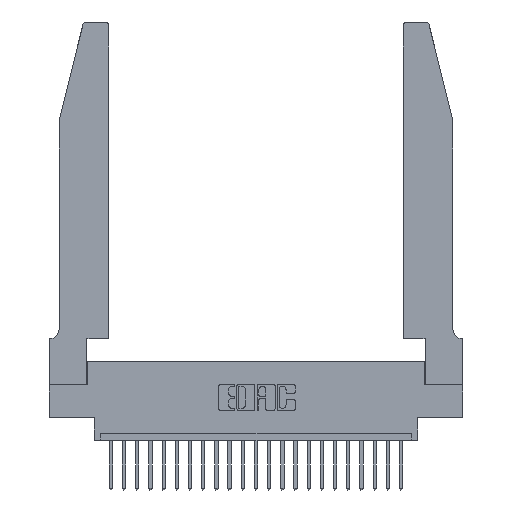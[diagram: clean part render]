
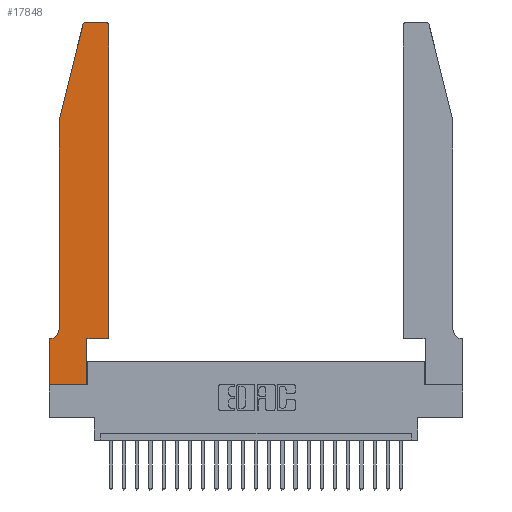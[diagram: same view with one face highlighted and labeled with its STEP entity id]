
A CAD part, top view. The second image highlights one B-rep face of the part: STEP entity #17848.
In plain terms, the highlighted planar face has unit normal (0, 0, 1).
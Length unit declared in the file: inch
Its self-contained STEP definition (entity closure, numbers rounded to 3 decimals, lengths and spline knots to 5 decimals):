
#230 = ORIENTED_EDGE ( 'NONE', *, *, #2061, .T. ) ;
#235 = EDGE_CURVE ( 'NONE', #24340, #12330, #18256, .T. ) ;
#681 = DIRECTION ( 'NONE',  ( 1., 0., 0. ) ) ;
#818 = ORIENTED_EDGE ( 'NONE', *, *, #8117, .T. ) ;
#1308 = CIRCLE ( 'NONE', #14758, 0.07 ) ;
#1358 = CARTESIAN_POINT ( 'NONE',  ( 0.0055, 0.35, 0.37 ) ) ;
#1642 = ORIENTED_EDGE ( 'NONE', *, *, #9878, .T. ) ;
#2061 = EDGE_CURVE ( 'NONE', #10363, #5751, #1308, .T. ) ;
#2111 = VECTOR ( 'NONE', #15944, 39.37008 ) ;
#2301 = VERTEX_POINT ( 'NONE', #24079 ) ;
#2437 = CARTESIAN_POINT ( 'NONE',  ( 0., 0., 0.37 ) ) ;
#2685 = EDGE_CURVE ( 'NONE', #10595, #16488, #19855, .T. ) ;
#3352 = CIRCLE ( 'NONE', #17424, 0.03 ) ;
#3377 = ORIENTED_EDGE ( 'NONE', *, *, #19977, .T. ) ;
#3501 = DIRECTION ( 'NONE',  ( 0., -1., 0. ) ) ;
#4023 = ORIENTED_EDGE ( 'NONE', *, *, #8189, .T. ) ;
#4123 = ORIENTED_EDGE ( 'NONE', *, *, #20316, .T. ) ;
#4272 = DIRECTION ( 'NONE',  ( 1., 0., 0. ) ) ;
#4963 = CARTESIAN_POINT ( 'NONE',  ( 0.0755, 0.35, 0.37 ) ) ;
#5459 = DIRECTION ( 'NONE',  ( -1., 0., 0. ) ) ;
#5542 = ORIENTED_EDGE ( 'NONE', *, *, #13575, .T. ) ;
#5706 = VECTOR ( 'NONE', #3501, 39.37008 ) ;
#5751 = VERTEX_POINT ( 'NONE', #1358 ) ;
#6104 = CARTESIAN_POINT ( 'NONE',  ( 0.4505, 0.35, 0.37 ) ) ;
#6284 = EDGE_CURVE ( 'NONE', #9132, #22724, #17614, .T. ) ;
#6970 = CARTESIAN_POINT ( 'NONE',  ( 0., 0.35, 0.37 ) ) ;
#6989 = CARTESIAN_POINT ( 'NONE',  ( 0.4505, 2.72, 0.37 ) ) ;
#7106 = VECTOR ( 'NONE', #9951, 39.37008 ) ;
#8117 = EDGE_CURVE ( 'NONE', #2301, #10363, #8726, .T. ) ;
#8189 = EDGE_CURVE ( 'NONE', #20644, #2301, #21287, .T. ) ;
#8279 = CARTESIAN_POINT ( 'NONE',  ( 0., 0.35, 0.37 ) ) ;
#8285 = CARTESIAN_POINT ( 'NONE',  ( 0.4505, 0.35, 0.37 ) ) ;
#8402 = LINE ( 'NONE', #8285, #13825 ) ;
#8407 = CARTESIAN_POINT ( 'NONE',  ( 0.284, 2.75, 0.37 ) ) ;
#8451 = CARTESIAN_POINT ( 'NONE',  ( 0.284, 2.72, 0.37 ) ) ;
#8726 = LINE ( 'NONE', #9552, #5706 ) ;
#8990 = EDGE_CURVE ( 'NONE', #16944, #9132, #8402, .T. ) ;
#9091 = EDGE_CURVE ( 'NONE', #14235, #10595, #19465, .T. ) ;
#9132 = VERTEX_POINT ( 'NONE', #18811 ) ;
#9552 = CARTESIAN_POINT ( 'NONE',  ( 0.0755, 2., 0.37 ) ) ;
#9878 = EDGE_CURVE ( 'NONE', #5751, #14235, #17365, .T. ) ;
#9919 = CARTESIAN_POINT ( 'NONE',  ( 0., 0., 0.37 ) ) ;
#9951 = DIRECTION ( 'NONE',  ( 0., 1., 0. ) ) ;
#10059 = DIRECTION ( 'NONE',  ( 1., 0., 0. ) ) ;
#10145 = DIRECTION ( 'NONE',  ( 0., 0., 1. ) ) ;
#10268 = LINE ( 'NONE', #23366, #11146 ) ;
#10363 = VERTEX_POINT ( 'NONE', #24070 ) ;
#10595 = VERTEX_POINT ( 'NONE', #9919 ) ;
#11146 = VECTOR ( 'NONE', #17612, 39.37008 ) ;
#11923 = ORIENTED_EDGE ( 'NONE', *, *, #2685, .T. ) ;
#11928 = CARTESIAN_POINT ( 'NONE',  ( 0.4205, 2.75, 0.37 ) ) ;
#11968 = CARTESIAN_POINT ( 'NONE',  ( 0.4205, 2.72, 0.37 ) ) ;
#12066 = DIRECTION ( 'NONE',  ( 1., 0., 0. ) ) ;
#12257 = VECTOR ( 'NONE', #14801, 39.37008 ) ;
#12330 = VERTEX_POINT ( 'NONE', #8407 ) ;
#12371 = CARTESIAN_POINT ( 'NONE',  ( 0.2865, 0.35, 0.37 ) ) ;
#13069 = CARTESIAN_POINT ( 'NONE',  ( 0.0755, 2., 0.37 ) ) ;
#13089 = ORIENTED_EDGE ( 'NONE', *, *, #6284, .T. ) ;
#13276 = CARTESIAN_POINT ( 'NONE',  ( 0.0055, 0.42, 0.37 ) ) ;
#13342 = AXIS2_PLACEMENT_3D ( 'NONE', #11968, #17530, #10059 ) ;
#13575 = EDGE_CURVE ( 'NONE', #12330, #20644, #3352, .T. ) ;
#13825 = VECTOR ( 'NONE', #12066, 39.37008 ) ;
#13862 = ORIENTED_EDGE ( 'NONE', *, *, #235, .T. ) ;
#14235 = VERTEX_POINT ( 'NONE', #8279 ) ;
#14758 = AXIS2_PLACEMENT_3D ( 'NONE', #13276, #15198, #5459 ) ;
#14801 = DIRECTION ( 'NONE',  ( -1., 0., 0. ) ) ;
#15113 = DIRECTION ( 'NONE',  ( -1., 0., 0. ) ) ;
#15198 = DIRECTION ( 'NONE',  ( 0., 0., -1. ) ) ;
#15680 = VECTOR ( 'NONE', #4272, 39.37008 ) ;
#15944 = DIRECTION ( 'NONE',  ( 0., -1., 0. ) ) ;
#16306 = ORIENTED_EDGE ( 'NONE', *, *, #8990, .T. ) ;
#16488 = VERTEX_POINT ( 'NONE', #22180 ) ;
#16944 = VERTEX_POINT ( 'NONE', #12371 ) ;
#17365 = LINE ( 'NONE', #4963, #12257 ) ;
#17424 = AXIS2_PLACEMENT_3D ( 'NONE', #8451, #10145, #681 ) ;
#17530 = DIRECTION ( 'NONE',  ( 0., 0., 1. ) ) ;
#17612 = DIRECTION ( 'NONE',  ( 0., 1., 0. ) ) ;
#17614 = LINE ( 'NONE', #6104, #7106 ) ;
#17848 = ADVANCED_FACE ( 'NONE', ( #18439 ), #18527, .T. ) ;
#18256 = LINE ( 'NONE', #22628, #18840 ) ;
#18418 = DIRECTION ( 'NONE',  ( -0.239, -0.971, 0. ) ) ;
#18439 = FACE_OUTER_BOUND ( 'NONE', #19154, .T. ) ;
#18491 = CARTESIAN_POINT ( 'NONE',  ( 0.25487, 2.72718, 0.37 ) ) ;
#18527 = PLANE ( 'NONE',  #23069 ) ;
#18811 = CARTESIAN_POINT ( 'NONE',  ( 0.4505, 0.35, 0.37 ) ) ;
#18840 = VECTOR ( 'NONE', #15113, 39.37008 ) ;
#18869 = VECTOR ( 'NONE', #18418, 39.37008 ) ;
#19154 = EDGE_LOOP ( 'NONE', ( #13862, #5542, #4023, #818, #230, #1642, #24623, #11923, #3377, #16306, #13089, #4123 ) ) ;
#19465 = LINE ( 'NONE', #19768, #2111 ) ;
#19768 = CARTESIAN_POINT ( 'NONE',  ( 0., 0., 0.37 ) ) ;
#19855 = LINE ( 'NONE', #2437, #15680 ) ;
#19977 = EDGE_CURVE ( 'NONE', #16488, #16944, #10268, .T. ) ;
#20316 = EDGE_CURVE ( 'NONE', #22724, #24340, #21023, .T. ) ;
#20559 = DIRECTION ( 'NONE',  ( 1., 0., 0. ) ) ;
#20644 = VERTEX_POINT ( 'NONE', #18491 ) ;
#21023 = CIRCLE ( 'NONE', #13342, 0.03 ) ;
#21287 = LINE ( 'NONE', #13069, #18869 ) ;
#22180 = CARTESIAN_POINT ( 'NONE',  ( 0.2865, 0., 0.37 ) ) ;
#22628 = CARTESIAN_POINT ( 'NONE',  ( 0.2605, 2.75, 0.37 ) ) ;
#22724 = VERTEX_POINT ( 'NONE', #6989 ) ;
#23069 = AXIS2_PLACEMENT_3D ( 'NONE', #6970, #24214, #20559 ) ;
#23366 = CARTESIAN_POINT ( 'NONE',  ( 0.2865, 0.35, 0.37 ) ) ;
#24070 = CARTESIAN_POINT ( 'NONE',  ( 0.0755, 0.42, 0.37 ) ) ;
#24079 = CARTESIAN_POINT ( 'NONE',  ( 0.0755, 2., 0.37 ) ) ;
#24214 = DIRECTION ( 'NONE',  ( 0., 0., 1. ) ) ;
#24340 = VERTEX_POINT ( 'NONE', #11928 ) ;
#24623 = ORIENTED_EDGE ( 'NONE', *, *, #9091, .T. ) ;
